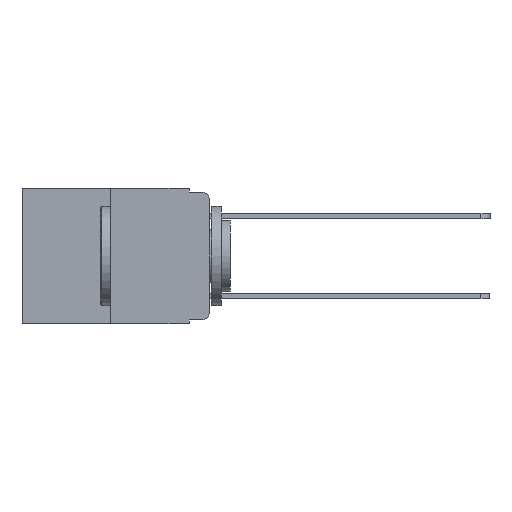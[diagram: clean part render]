
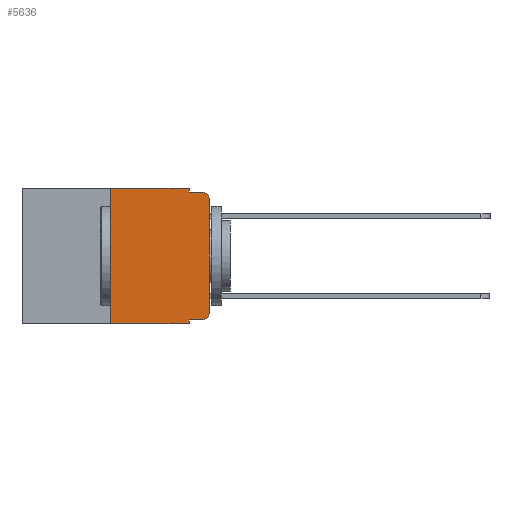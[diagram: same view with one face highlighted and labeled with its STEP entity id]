
A CAD part, left-side view. The second image highlights one B-rep face of the part: STEP entity #5636.
In plain terms, the highlighted planar face has unit normal (-1, 0, 0).
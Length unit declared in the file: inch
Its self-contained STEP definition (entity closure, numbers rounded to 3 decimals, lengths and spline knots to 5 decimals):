
#134 = EDGE_CURVE ( 'NONE', #4793, #8488, #293, .T. ) ;
#293 = CIRCLE ( 'NONE', #14125, 0.02 ) ;
#556 = CARTESIAN_POINT ( 'NONE',  ( 0., 0.051, -0.343 ) ) ;
#616 = ORIENTED_EDGE ( 'NONE', *, *, #5513, .F. ) ;
#753 = VERTEX_POINT ( 'NONE', #556 ) ;
#945 = CARTESIAN_POINT ( 'NONE',  ( 0., 0.02, -0.333 ) ) ;
#1017 = DIRECTION ( 'NONE',  ( 0., 0., -1. ) ) ;
#1162 = VERTEX_POINT ( 'NONE', #945 ) ;
#1242 = PLANE ( 'NONE',  #14430 ) ;
#1576 = CARTESIAN_POINT ( 'NONE',  ( 0., 0.051, -0.01 ) ) ;
#1783 = CARTESIAN_POINT ( 'NONE',  ( 0., 0.051, -0.333 ) ) ;
#2422 = CARTESIAN_POINT ( 'NONE',  ( 0., 0., -0.313 ) ) ;
#2626 = CARTESIAN_POINT ( 'NONE',  ( 0., 0.473, 0. ) ) ;
#2671 = LINE ( 'NONE', #8723, #5825 ) ;
#2697 = VERTEX_POINT ( 'NONE', #2422 ) ;
#2746 = DIRECTION ( 'NONE',  ( 0., 0., -1. ) ) ;
#3158 = DIRECTION ( 'NONE',  ( 0., -1., 0. ) ) ;
#3205 = LINE ( 'NONE', #10028, #16190 ) ;
#3241 = ORIENTED_EDGE ( 'NONE', *, *, #14182, .T. ) ;
#3590 = DIRECTION ( 'NONE',  ( 0., -1., 0. ) ) ;
#4490 = ORIENTED_EDGE ( 'NONE', *, *, #13446, .F. ) ;
#4526 = ORIENTED_EDGE ( 'NONE', *, *, #10150, .T. ) ;
#4793 = VERTEX_POINT ( 'NONE', #4866 ) ;
#4866 = CARTESIAN_POINT ( 'NONE',  ( 0., 0., -0.03 ) ) ;
#5396 = LINE ( 'NONE', #1783, #11721 ) ;
#5482 = VERTEX_POINT ( 'NONE', #9862 ) ;
#5513 = EDGE_CURVE ( 'NONE', #11957, #5482, #9330, .T. ) ;
#5635 = VERTEX_POINT ( 'NONE', #12835 ) ;
#5636 = ADVANCED_FACE ( 'NONE', ( #15420 ), #1242, .F. ) ;
#5825 = VECTOR ( 'NONE', #12368, 39.37008 ) ;
#5851 = CARTESIAN_POINT ( 'NONE',  ( 0., 0.25, 0. ) ) ;
#6582 = CARTESIAN_POINT ( 'NONE',  ( 0., 0.02, -0.01 ) ) ;
#6638 = CARTESIAN_POINT ( 'NONE',  ( 0., 0.02, -0.03 ) ) ;
#6640 = VERTEX_POINT ( 'NONE', #1576 ) ;
#6659 = DIRECTION ( 'NONE',  ( -1., 0., 0. ) ) ;
#6856 = ORIENTED_EDGE ( 'NONE', *, *, #11014, .T. ) ;
#7407 = ORIENTED_EDGE ( 'NONE', *, *, #134, .T. ) ;
#7516 = DIRECTION ( 'NONE',  ( 0., -1., 0. ) ) ;
#7559 = VECTOR ( 'NONE', #7516, 39.37008 ) ;
#7577 = VECTOR ( 'NONE', #10300, 39.37008 ) ;
#8474 = ORIENTED_EDGE ( 'NONE', *, *, #14285, .F. ) ;
#8488 = VERTEX_POINT ( 'NONE', #6582 ) ;
#8723 = CARTESIAN_POINT ( 'NONE',  ( 0., 0., 0. ) ) ;
#8972 = DIRECTION ( 'NONE',  ( -1., 0., 0. ) ) ;
#9017 = CARTESIAN_POINT ( 'NONE',  ( 0., 0.051, 0. ) ) ;
#9279 = ORIENTED_EDGE ( 'NONE', *, *, #15903, .T. ) ;
#9330 = LINE ( 'NONE', #12203, #12542 ) ;
#9862 = CARTESIAN_POINT ( 'NONE',  ( 0., 0.051, 0. ) ) ;
#9947 = VECTOR ( 'NONE', #11453, 39.37008 ) ;
#10028 = CARTESIAN_POINT ( 'NONE',  ( 0., 0.051, 0. ) ) ;
#10148 = AXIS2_PLACEMENT_3D ( 'NONE', #16235, #8972, #1017 ) ;
#10150 = EDGE_CURVE ( 'NONE', #1162, #2697, #12092, .T. ) ;
#10300 = DIRECTION ( 'NONE',  ( 0., 0., 1. ) ) ;
#10308 = VERTEX_POINT ( 'NONE', #15162 ) ;
#10490 = DIRECTION ( 'NONE',  ( 1., 0., 0. ) ) ;
#11014 = EDGE_CURVE ( 'NONE', #10308, #1162, #5396, .T. ) ;
#11175 = VECTOR ( 'NONE', #13691, 39.37008 ) ;
#11369 = DIRECTION ( 'NONE',  ( 0., 0., -1. ) ) ;
#11453 = DIRECTION ( 'NONE',  ( 0., 0., -1. ) ) ;
#11549 = LINE ( 'NONE', #14907, #11175 ) ;
#11721 = VECTOR ( 'NONE', #3158, 39.37008 ) ;
#11957 = VERTEX_POINT ( 'NONE', #5851 ) ;
#12092 = CIRCLE ( 'NONE', #10148, 0.02 ) ;
#12203 = CARTESIAN_POINT ( 'NONE',  ( 0., 0.473, 0. ) ) ;
#12340 = ORIENTED_EDGE ( 'NONE', *, *, #15091, .F. ) ;
#12368 = DIRECTION ( 'NONE',  ( 0., 0., 1. ) ) ;
#12422 = CARTESIAN_POINT ( 'NONE',  ( 0., 0.473, -0.343 ) ) ;
#12542 = VECTOR ( 'NONE', #3590, 39.37008 ) ;
#12608 = EDGE_CURVE ( 'NONE', #10308, #753, #13204, .T. ) ;
#12609 = EDGE_LOOP ( 'NONE', ( #9279, #7407, #12340, #8474, #616, #4490, #3241, #14393, #6856, #4526 ) ) ;
#12835 = CARTESIAN_POINT ( 'NONE',  ( 0., 0.25, -0.343 ) ) ;
#13204 = LINE ( 'NONE', #9017, #9947 ) ;
#13446 = EDGE_CURVE ( 'NONE', #5635, #11957, #14142, .T. ) ;
#13691 = DIRECTION ( 'NONE',  ( 0., -1., 0. ) ) ;
#14125 = AXIS2_PLACEMENT_3D ( 'NONE', #6638, #6659, #14674 ) ;
#14142 = LINE ( 'NONE', #15241, #7577 ) ;
#14182 = EDGE_CURVE ( 'NONE', #5635, #753, #14890, .T. ) ;
#14285 = EDGE_CURVE ( 'NONE', #5482, #6640, #3205, .T. ) ;
#14393 = ORIENTED_EDGE ( 'NONE', *, *, #12608, .F. ) ;
#14430 = AXIS2_PLACEMENT_3D ( 'NONE', #2626, #10490, #2746 ) ;
#14674 = DIRECTION ( 'NONE',  ( 0., 0., -1. ) ) ;
#14890 = LINE ( 'NONE', #12422, #7559 ) ;
#14907 = CARTESIAN_POINT ( 'NONE',  ( 0., 0.051, -0.01 ) ) ;
#15091 = EDGE_CURVE ( 'NONE', #6640, #8488, #11549, .T. ) ;
#15162 = CARTESIAN_POINT ( 'NONE',  ( 0., 0.051, -0.333 ) ) ;
#15241 = CARTESIAN_POINT ( 'NONE',  ( 0., 0.25, 0. ) ) ;
#15420 = FACE_OUTER_BOUND ( 'NONE', #12609, .T. ) ;
#15903 = EDGE_CURVE ( 'NONE', #2697, #4793, #2671, .T. ) ;
#16190 = VECTOR ( 'NONE', #11369, 39.37008 ) ;
#16235 = CARTESIAN_POINT ( 'NONE',  ( 0., 0.02, -0.313 ) ) ;
